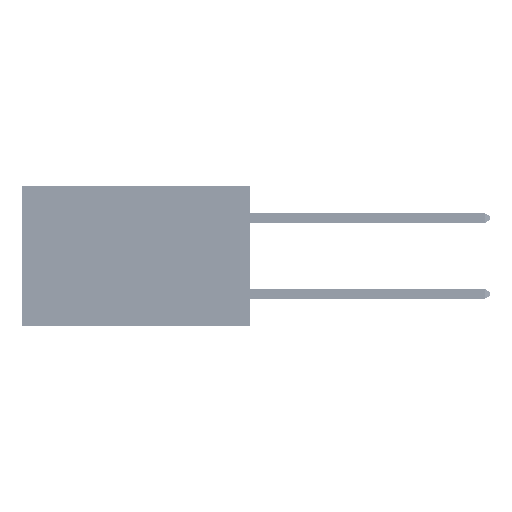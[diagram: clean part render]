
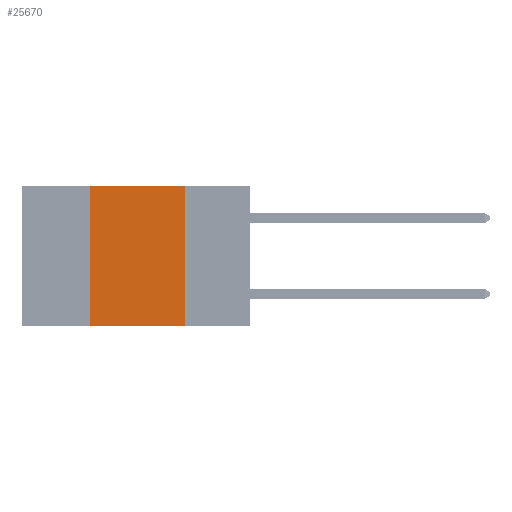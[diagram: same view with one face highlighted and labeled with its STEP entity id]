
A CAD part, left-side view. The second image highlights one B-rep face of the part: STEP entity #25670.
In plain terms, the highlighted planar face has unit normal (-1, 0, 0).
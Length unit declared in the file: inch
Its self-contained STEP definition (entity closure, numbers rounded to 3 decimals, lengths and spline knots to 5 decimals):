
#644 = FACE_OUTER_BOUND ( 'NONE', #1525, .T. ) ;
#1525 = EDGE_LOOP ( 'NONE', ( #28446, #48591, #46469, #28622 ) ) ;
#1825 = EDGE_CURVE ( 'NONE', #46999, #14193, #29393, .T. ) ;
#4323 = CARTESIAN_POINT ( 'NONE',  ( 0., 0.42, 0. ) ) ;
#4431 = DIRECTION ( 'NONE',  ( 1., 0., 0. ) ) ;
#4750 = DIRECTION ( 'NONE',  ( 0., 0., -1. ) ) ;
#4970 = DIRECTION ( 'NONE',  ( 0., 0., 1. ) ) ;
#7049 = VECTOR ( 'NONE', #25118, 39.37008 ) ;
#7577 = EDGE_CURVE ( 'NONE', #46999, #17181, #40332, .T. ) ;
#10527 = VECTOR ( 'NONE', #33305, 39.37008 ) ;
#11009 = CARTESIAN_POINT ( 'NONE',  ( 0., 0.17, 0. ) ) ;
#11804 = PLANE ( 'NONE',  #45400 ) ;
#12145 = CARTESIAN_POINT ( 'NONE',  ( 0., 0.6, 0. ) ) ;
#14193 = VERTEX_POINT ( 'NONE', #41100 ) ;
#17181 = VERTEX_POINT ( 'NONE', #35438 ) ;
#18554 = VECTOR ( 'NONE', #4970, 39.37008 ) ;
#21326 = VECTOR ( 'NONE', #37822, 39.37008 ) ;
#24329 = EDGE_CURVE ( 'NONE', #30264, #14193, #37824, .T. ) ;
#25118 = DIRECTION ( 'NONE',  ( 0., -1., 0. ) ) ;
#25670 = ADVANCED_FACE ( 'NONE', ( #644 ), #11804, .F. ) ;
#28446 = ORIENTED_EDGE ( 'NONE', *, *, #24329, .F. ) ;
#28622 = ORIENTED_EDGE ( 'NONE', *, *, #1825, .T. ) ;
#29393 = LINE ( 'NONE', #35524, #7049 ) ;
#29671 = CARTESIAN_POINT ( 'NONE',  ( 0., 0.6, 0. ) ) ;
#30264 = VERTEX_POINT ( 'NONE', #35337 ) ;
#31701 = LINE ( 'NONE', #29671, #10527 ) ;
#31722 = CARTESIAN_POINT ( 'NONE',  ( 0., 0.42, -0.37 ) ) ;
#33305 = DIRECTION ( 'NONE',  ( 0., -1., 0. ) ) ;
#35337 = CARTESIAN_POINT ( 'NONE',  ( 0., 0.17, 0. ) ) ;
#35438 = CARTESIAN_POINT ( 'NONE',  ( 0., 0.42, 0. ) ) ;
#35524 = CARTESIAN_POINT ( 'NONE',  ( 0., 0.6, -0.37 ) ) ;
#37822 = DIRECTION ( 'NONE',  ( 0., 0., -1. ) ) ;
#37824 = LINE ( 'NONE', #11009, #21326 ) ;
#39788 = EDGE_CURVE ( 'NONE', #17181, #30264, #31701, .T. ) ;
#40332 = LINE ( 'NONE', #4323, #18554 ) ;
#41100 = CARTESIAN_POINT ( 'NONE',  ( 0., 0.17, -0.37 ) ) ;
#45400 = AXIS2_PLACEMENT_3D ( 'NONE', #12145, #4431, #4750 ) ;
#46469 = ORIENTED_EDGE ( 'NONE', *, *, #7577, .F. ) ;
#46999 = VERTEX_POINT ( 'NONE', #31722 ) ;
#48591 = ORIENTED_EDGE ( 'NONE', *, *, #39788, .F. ) ;
